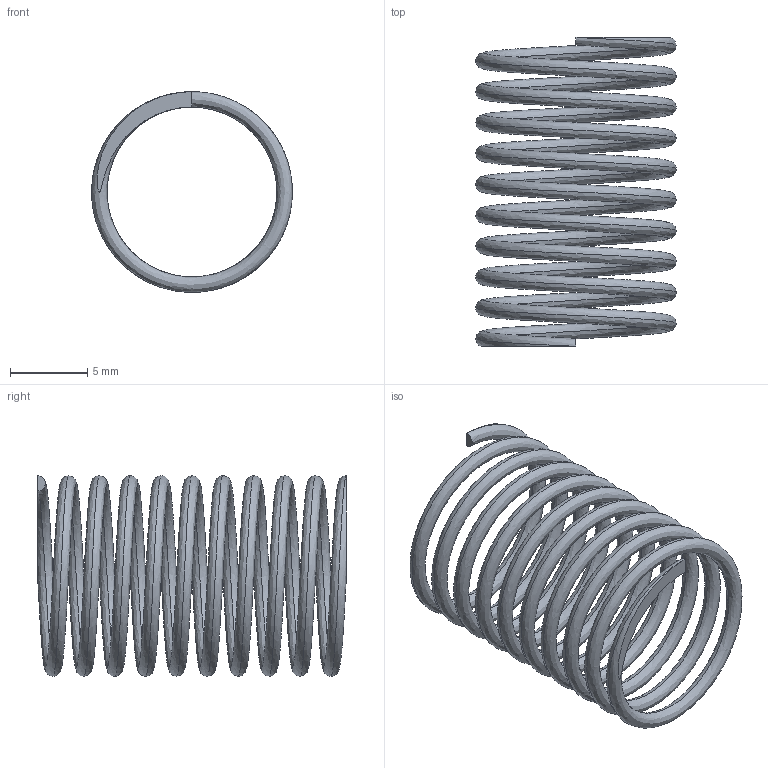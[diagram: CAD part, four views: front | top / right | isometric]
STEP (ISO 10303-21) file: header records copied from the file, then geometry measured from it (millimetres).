
FILE_DESCRIPTION (( 'STEP AP214' ), '1' );
FILE_NAME ('key_spring.STEP', '2013-12-22T02:52:09', ( '' ), ( '' ), 'SwSTEP 2.0', 'SolidWorks 2013', '' );
FILE_SCHEMA (( 'AUTOMOTIVE_DESIGN' ));
Length unit declared in the file: millimetre
Products named in the file (1): key_spring
Bounding box: 13 x 20 x 13 mm (x, y, z)
Volume: 293.1 mm3; surface area: 1182.1 mm2
Topology: 1 solids, 1 shells, 6 faces, 8 edges, 4 vertices
Faces by surface type: plane 4, bspline 2
Entity records: 3463 total; most frequent: CARTESIAN_POINT 3344, DIRECTION 16, ORIENTED_EDGE 16, EDGE_CURVE 8, AXIS2_PLACEMENT_3D 7, EDGE_LOOP 6, ADVANCED_FACE 6, FACE_OUTER_BOUND 6
